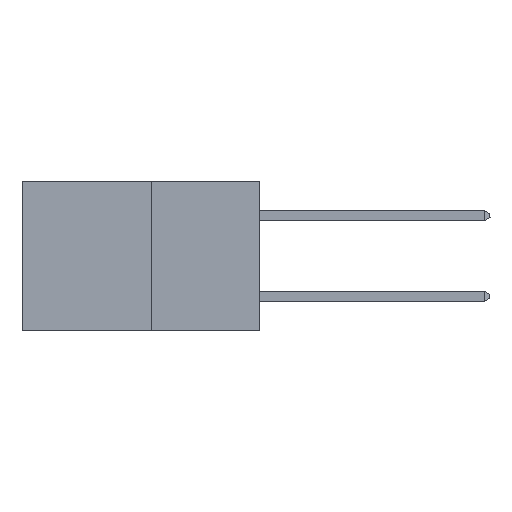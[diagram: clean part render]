
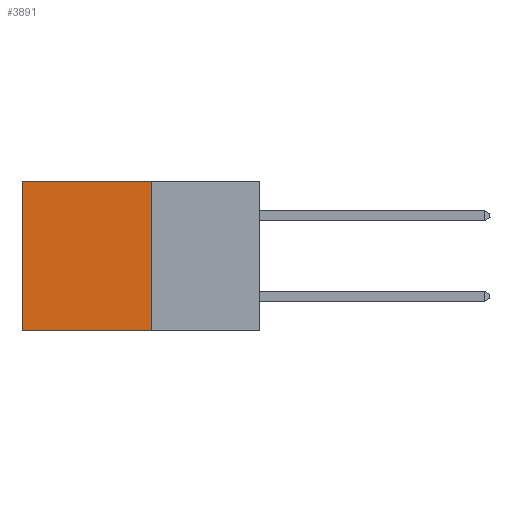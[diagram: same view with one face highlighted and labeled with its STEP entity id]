
A CAD part, left-side view. The second image highlights one B-rep face of the part: STEP entity #3891.
In plain terms, the highlighted planar face has unit normal (-1, 0, 0).
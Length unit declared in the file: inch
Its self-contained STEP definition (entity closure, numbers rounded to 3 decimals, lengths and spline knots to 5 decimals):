
#77 = EDGE_CURVE ( 'NONE', #5682, #2068, #11843, .T. ) ;
#1806 = VERTEX_POINT ( 'NONE', #14036 ) ;
#2068 = VERTEX_POINT ( 'NONE', #7137 ) ;
#2092 = DIRECTION ( 'NONE',  ( 0., 1., 0. ) ) ;
#2107 = DIRECTION ( 'NONE',  ( 0., 0., -1. ) ) ;
#2763 = DIRECTION ( 'NONE',  ( 1., 0., 0. ) ) ;
#2862 = AXIS2_PLACEMENT_3D ( 'NONE', #15649, #2763, #11853 ) ;
#3449 = VECTOR ( 'NONE', #6972, 39.37008 ) ;
#3848 = VECTOR ( 'NONE', #8518, 39.37008 ) ;
#3891 = ADVANCED_FACE ( 'NONE', ( #8826 ), #10546, .F. ) ;
#4263 = VERTEX_POINT ( 'NONE', #7503 ) ;
#4558 = CARTESIAN_POINT ( 'NONE',  ( 0.277, 0.27, 0. ) ) ;
#4952 = VECTOR ( 'NONE', #2092, 39.37008 ) ;
#5682 = VERTEX_POINT ( 'NONE', #7786 ) ;
#6033 = EDGE_LOOP ( 'NONE', ( #15047, #11964, #13069, #7519 ) ) ;
#6127 = VECTOR ( 'NONE', #2107, 39.37008 ) ;
#6733 = EDGE_CURVE ( 'NONE', #1806, #4263, #14558, .T. ) ;
#6811 = EDGE_CURVE ( 'NONE', #4263, #2068, #16331, .T. ) ;
#6972 = DIRECTION ( 'NONE',  ( 0., 0., -1. ) ) ;
#7137 = CARTESIAN_POINT ( 'NONE',  ( 0.277, 0.59, -0.37 ) ) ;
#7503 = CARTESIAN_POINT ( 'NONE',  ( 0.277, 0.59, 0. ) ) ;
#7519 = ORIENTED_EDGE ( 'NONE', *, *, #6733, .T. ) ;
#7786 = CARTESIAN_POINT ( 'NONE',  ( 0.277, 0.27, -0.37 ) ) ;
#8234 = CARTESIAN_POINT ( 'NONE',  ( 0.277, 0.27, -0.37 ) ) ;
#8518 = DIRECTION ( 'NONE',  ( 0., 1., 0. ) ) ;
#8826 = FACE_OUTER_BOUND ( 'NONE', #6033, .T. ) ;
#10546 = PLANE ( 'NONE',  #2862 ) ;
#11163 = CARTESIAN_POINT ( 'NONE',  ( 0.277, 0.59, -0.37 ) ) ;
#11549 = EDGE_CURVE ( 'NONE', #1806, #5682, #13788, .T. ) ;
#11843 = LINE ( 'NONE', #14699, #4952 ) ;
#11853 = DIRECTION ( 'NONE',  ( 0., 0., -1. ) ) ;
#11964 = ORIENTED_EDGE ( 'NONE', *, *, #77, .F. ) ;
#13069 = ORIENTED_EDGE ( 'NONE', *, *, #11549, .F. ) ;
#13788 = LINE ( 'NONE', #8234, #3449 ) ;
#14036 = CARTESIAN_POINT ( 'NONE',  ( 0.277, 0.27, 0. ) ) ;
#14558 = LINE ( 'NONE', #4558, #3848 ) ;
#14699 = CARTESIAN_POINT ( 'NONE',  ( 0.277, 0.27, -0.37 ) ) ;
#15047 = ORIENTED_EDGE ( 'NONE', *, *, #6811, .T. ) ;
#15649 = CARTESIAN_POINT ( 'NONE',  ( 0.277, 0.27, -0.37 ) ) ;
#16331 = LINE ( 'NONE', #11163, #6127 ) ;
